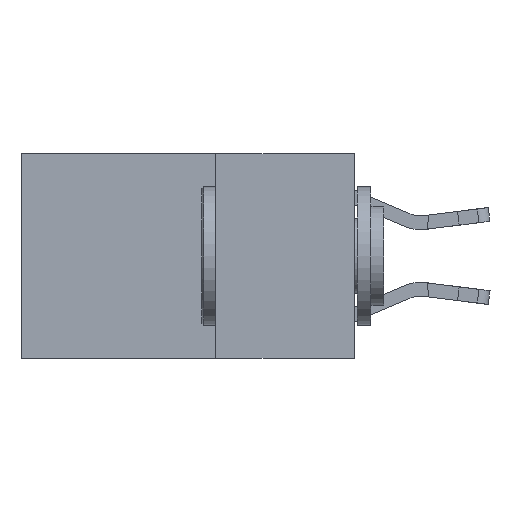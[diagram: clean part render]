
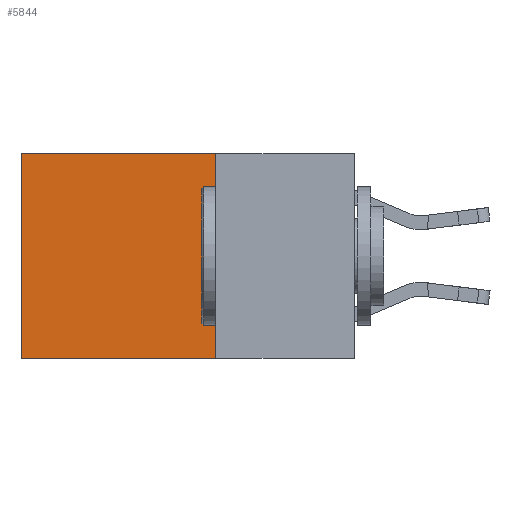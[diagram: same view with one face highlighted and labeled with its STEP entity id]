
A CAD part, left-side view. The second image highlights one B-rep face of the part: STEP entity #5844.
In plain terms, the highlighted planar face has unit normal (-1, 0, 0).
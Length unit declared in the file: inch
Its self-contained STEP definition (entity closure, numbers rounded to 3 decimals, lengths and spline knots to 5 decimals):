
#227 = CARTESIAN_POINT ( 'NONE',  ( 0.2625, 0.25, -0.37 ) ) ;
#887 = VECTOR ( 'NONE', #2395, 39.37008 ) ;
#917 = EDGE_CURVE ( 'NONE', #3166, #978, #4759, .T. ) ;
#978 = VERTEX_POINT ( 'NONE', #2000 ) ;
#1355 = CARTESIAN_POINT ( 'NONE',  ( 0.2625, 0.6, 0. ) ) ;
#1809 = VECTOR ( 'NONE', #3052, 39.37008 ) ;
#1987 = VERTEX_POINT ( 'NONE', #4174 ) ;
#2000 = CARTESIAN_POINT ( 'NONE',  ( 0.2625, 0.6, -0.37 ) ) ;
#2012 = CARTESIAN_POINT ( 'NONE',  ( 0.2625, 0.25, 0. ) ) ;
#2082 = VECTOR ( 'NONE', #7807, 39.37008 ) ;
#2185 = DIRECTION ( 'NONE',  ( 0., 1., 0. ) ) ;
#2395 = DIRECTION ( 'NONE',  ( 0., 0., -1. ) ) ;
#2500 = ORIENTED_EDGE ( 'NONE', *, *, #3314, .T. ) ;
#2811 = ORIENTED_EDGE ( 'NONE', *, *, #3718, .F. ) ;
#2947 = CARTESIAN_POINT ( 'NONE',  ( 0.2625, 0.25, -0.37 ) ) ;
#3052 = DIRECTION ( 'NONE',  ( 0., 0., -1. ) ) ;
#3166 = VERTEX_POINT ( 'NONE', #227 ) ;
#3177 = VERTEX_POINT ( 'NONE', #8147 ) ;
#3314 = EDGE_CURVE ( 'NONE', #3177, #978, #8995, .T. ) ;
#3718 = EDGE_CURVE ( 'NONE', #1987, #3166, #4495, .T. ) ;
#4090 = LINE ( 'NONE', #8049, #6067 ) ;
#4174 = CARTESIAN_POINT ( 'NONE',  ( 0.2625, 0.25, 0. ) ) ;
#4495 = LINE ( 'NONE', #2012, #1809 ) ;
#4759 = LINE ( 'NONE', #2947, #2082 ) ;
#4917 = DIRECTION ( 'NONE',  ( 0., 0., -1. ) ) ;
#5146 = ORIENTED_EDGE ( 'NONE', *, *, #917, .F. ) ;
#5844 = ADVANCED_FACE ( 'NONE', ( #11715 ), #8717, .F. ) ;
#6067 = VECTOR ( 'NONE', #2185, 39.37008 ) ;
#6754 = AXIS2_PLACEMENT_3D ( 'NONE', #9664, #10605, #4917 ) ;
#7398 = EDGE_LOOP ( 'NONE', ( #2500, #5146, #2811, #10493 ) ) ;
#7807 = DIRECTION ( 'NONE',  ( 0., 1., 0. ) ) ;
#8049 = CARTESIAN_POINT ( 'NONE',  ( 0.2625, 0.25, 0. ) ) ;
#8147 = CARTESIAN_POINT ( 'NONE',  ( 0.2625, 0.6, 0. ) ) ;
#8717 = PLANE ( 'NONE',  #6754 ) ;
#8995 = LINE ( 'NONE', #1355, #887 ) ;
#9664 = CARTESIAN_POINT ( 'NONE',  ( 0.2625, 0.25, 0. ) ) ;
#10493 = ORIENTED_EDGE ( 'NONE', *, *, #10631, .T. ) ;
#10605 = DIRECTION ( 'NONE',  ( 1., 0., 0. ) ) ;
#10631 = EDGE_CURVE ( 'NONE', #1987, #3177, #4090, .T. ) ;
#11715 = FACE_OUTER_BOUND ( 'NONE', #7398, .T. ) ;
